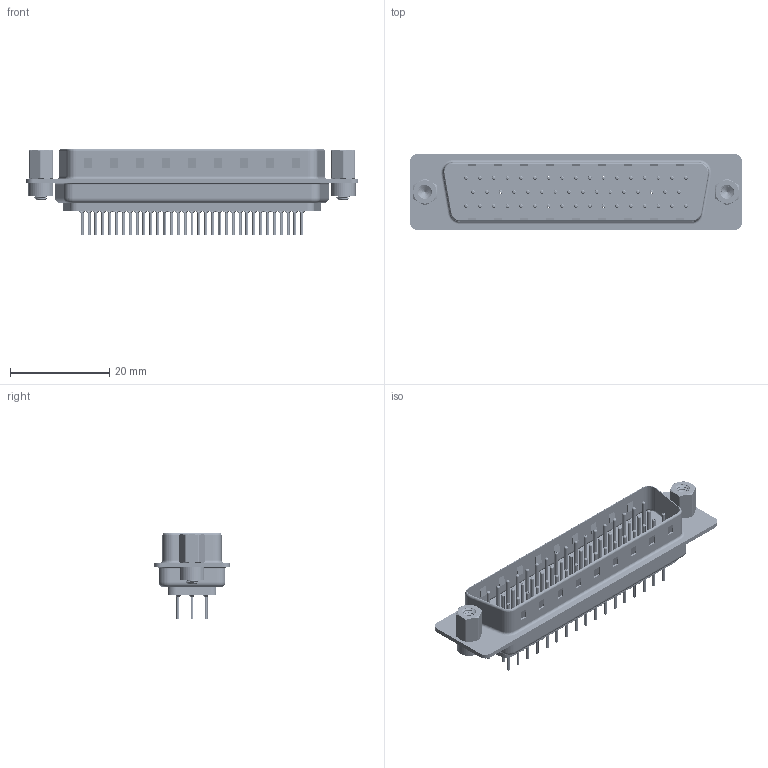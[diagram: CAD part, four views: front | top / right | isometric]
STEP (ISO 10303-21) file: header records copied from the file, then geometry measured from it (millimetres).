
FILE_DESCRIPTION (( 'STEP AP203' ), '1' );
FILE_NAME ('627-050-620-263.STEP', '2020-07-15T15:29:02', ( '' ), ( '' ), 'SwSTEP 2.0', 'SolidWorks 2020', '' );
FILE_SCHEMA (( 'CONFIG_CONTROL_DESIGN' ));
Length unit declared in the file: millimetre
Products named in the file (9): 627 Housing_50 LP; 627 4-40 Threaded Rivet; 627 Contact Row 2_20L; 627 Shell Front_50 Contacts; 627 Contact Row 1_20L; 627 Contact Row 3_20L; 627 4-40 Hex Standoff; 627-050-620-263; 627 Shell Rear_50 Contacts
Assembly tree (57 placements, depth 2):
  627-050-620-263
    627 Housing_50 LP
    627 Shell Front_50 Contacts
    627 Shell Rear_50 Contacts
    627 Contact Row 1_20L  x17
    627 Contact Row 2_20L  x16
    627 Contact Row 3_20L  x17
    627 4-40 Threaded Rivet  x2
    627 4-40 Hex Standoff  x2
Bounding box: 67 x 15.3 x 17.3 mm (x, y, z)
Volume: 4631.3 mm3; surface area: 13056.6 mm2
Topology: 57 solids, 57 shells, 5434 faces, 14245 edges, 8836 vertices
Faces by surface type: cylinder 2061, plane 1425, torus 1400, cone 530, bspline 18
Entity records: 40659 total; most frequent: CARTESIAN_POINT 10893, DIRECTION 6130, ORIENTED_EDGE 5496, EDGE_CURVE 2748, AXIS2_PLACEMENT_3D 2453, VERTEX_POINT 1765, EDGE_LOOP 1371, CIRCLE 1292
